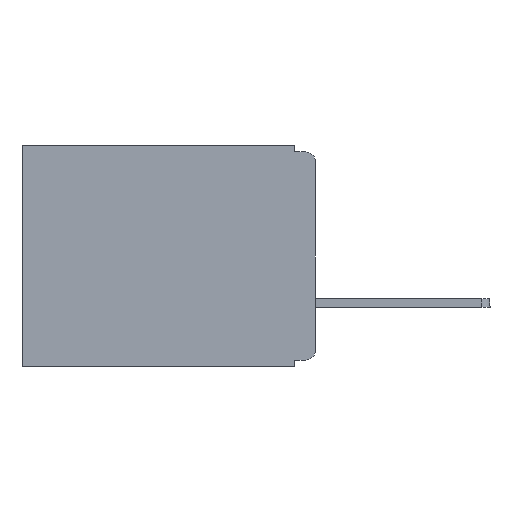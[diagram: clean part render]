
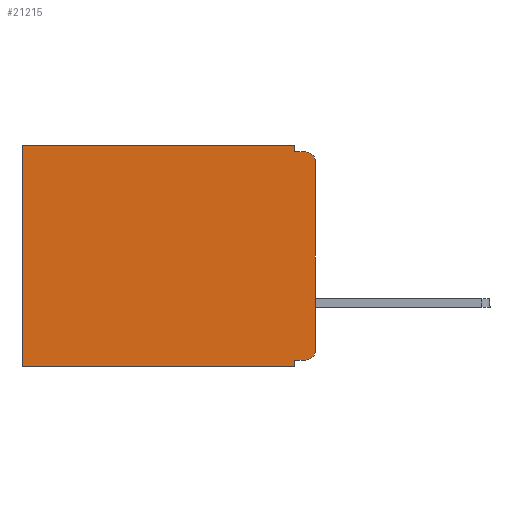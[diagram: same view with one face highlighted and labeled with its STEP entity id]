
A CAD part, left-side view. The second image highlights one B-rep face of the part: STEP entity #21215.
In plain terms, the highlighted planar face has unit normal (-1, 0, 0).
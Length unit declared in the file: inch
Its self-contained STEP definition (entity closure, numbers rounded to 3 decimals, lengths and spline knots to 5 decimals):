
#140 = VECTOR ( 'NONE', #14403, 39.37008 ) ;
#962 = FACE_OUTER_BOUND ( 'NONE', #12624, .T. ) ;
#1121 = VECTOR ( 'NONE', #1252, 39.37008 ) ;
#1252 = DIRECTION ( 'NONE',  ( 0., 0., -1. ) ) ;
#1561 = ORIENTED_EDGE ( 'NONE', *, *, #5486, .F. ) ;
#1730 = CARTESIAN_POINT ( 'NONE',  ( 0.3, 0.031, -0.33 ) ) ;
#2026 = CARTESIAN_POINT ( 'NONE',  ( 0.3, 0.015, -0.305 ) ) ;
#2272 = CARTESIAN_POINT ( 'NONE',  ( 0.3, 0., -0.33 ) ) ;
#2291 = DIRECTION ( 'NONE',  ( 0., 0., -1. ) ) ;
#2718 = CIRCLE ( 'NONE', #22640, 0.015 ) ;
#2800 = CARTESIAN_POINT ( 'NONE',  ( 0.3, 0., -0.33 ) ) ;
#3053 = DIRECTION ( 'NONE',  ( 0., -1., 0. ) ) ;
#3244 = CARTESIAN_POINT ( 'NONE',  ( 0.3, 0., -0.33 ) ) ;
#3465 = ORIENTED_EDGE ( 'NONE', *, *, #17571, .T. ) ;
#3485 = CARTESIAN_POINT ( 'NONE',  ( 0.3, 0.437, -0.33 ) ) ;
#3636 = EDGE_CURVE ( 'NONE', #11892, #8520, #13092, .T. ) ;
#3879 = VERTEX_POINT ( 'NONE', #6805 ) ;
#3928 = ORIENTED_EDGE ( 'NONE', *, *, #9904, .F. ) ;
#3989 = DIRECTION ( 'NONE',  ( 0., 0., -1. ) ) ;
#4638 = EDGE_CURVE ( 'NONE', #15721, #8520, #15747, .T. ) ;
#5136 = CARTESIAN_POINT ( 'NONE',  ( 0.3, 0.031, -0.32 ) ) ;
#5183 = CARTESIAN_POINT ( 'NONE',  ( 0.3, 0.031, -0.01 ) ) ;
#5215 = DIRECTION ( 'NONE',  ( 0., 0., -1. ) ) ;
#5486 = EDGE_CURVE ( 'NONE', #11892, #22754, #9276, .T. ) ;
#5945 = CARTESIAN_POINT ( 'NONE',  ( 0.3, 0.437, -0.33 ) ) ;
#6805 = CARTESIAN_POINT ( 'NONE',  ( 0.3, 0.015, -0.32 ) ) ;
#6896 = VERTEX_POINT ( 'NONE', #5136 ) ;
#6930 = ORIENTED_EDGE ( 'NONE', *, *, #13381, .F. ) ;
#7332 = LINE ( 'NONE', #24920, #17737 ) ;
#7629 = CARTESIAN_POINT ( 'NONE',  ( 0.3, 0.031, 0. ) ) ;
#7677 = CARTESIAN_POINT ( 'NONE',  ( 0.3, 0., -0.01 ) ) ;
#8383 = CARTESIAN_POINT ( 'NONE',  ( 0.3, 0.015, -0.01 ) ) ;
#8484 = AXIS2_PLACEMENT_3D ( 'NONE', #3244, #16938, #5215 ) ;
#8520 = VERTEX_POINT ( 'NONE', #8383 ) ;
#9276 = LINE ( 'NONE', #2272, #14460 ) ;
#9584 = ORIENTED_EDGE ( 'NONE', *, *, #16401, .T. ) ;
#9593 = DIRECTION ( 'NONE',  ( 0., 0., -1. ) ) ;
#9713 = VERTEX_POINT ( 'NONE', #5945 ) ;
#9904 = EDGE_CURVE ( 'NONE', #3879, #6896, #20897, .T. ) ;
#10263 = ORIENTED_EDGE ( 'NONE', *, *, #23991, .F. ) ;
#10330 = VECTOR ( 'NONE', #13284, 39.37008 ) ;
#11076 = ORIENTED_EDGE ( 'NONE', *, *, #4638, .F. ) ;
#11211 = CARTESIAN_POINT ( 'NONE',  ( 0.3, 0.015, -0.025 ) ) ;
#11425 = DIRECTION ( 'NONE',  ( 0., 1., 0. ) ) ;
#11566 = LINE ( 'NONE', #3485, #10330 ) ;
#11892 = VERTEX_POINT ( 'NONE', #17041 ) ;
#12520 = DIRECTION ( 'NONE',  ( -1., 0., 0. ) ) ;
#12586 = DIRECTION ( 'NONE',  ( 0., 0., -1. ) ) ;
#12609 = EDGE_CURVE ( 'NONE', #3879, #22754, #2718, .T. ) ;
#12624 = EDGE_LOOP ( 'NONE', ( #1561, #21098, #11076, #19906, #9584, #3465, #6930, #10263, #3928, #22534 ) ) ;
#13092 = CIRCLE ( 'NONE', #24223, 0.015 ) ;
#13099 = VECTOR ( 'NONE', #9593, 39.37008 ) ;
#13284 = DIRECTION ( 'NONE',  ( 0., 0., -1. ) ) ;
#13357 = LINE ( 'NONE', #7629, #13099 ) ;
#13381 = EDGE_CURVE ( 'NONE', #16997, #9713, #23982, .T. ) ;
#14403 = DIRECTION ( 'NONE',  ( 0., 1., 0. ) ) ;
#14460 = VECTOR ( 'NONE', #2291, 39.37008 ) ;
#14916 = CARTESIAN_POINT ( 'NONE',  ( 0.3, 0.031, -0.33 ) ) ;
#15111 = VECTOR ( 'NONE', #3053, 39.37008 ) ;
#15575 = VERTEX_POINT ( 'NONE', #18424 ) ;
#15692 = DIRECTION ( 'NONE',  ( -1., 0., 0. ) ) ;
#15721 = VERTEX_POINT ( 'NONE', #5183 ) ;
#15747 = LINE ( 'NONE', #7677, #15111 ) ;
#16401 = EDGE_CURVE ( 'NONE', #15575, #21978, #7332, .T. ) ;
#16508 = DIRECTION ( 'NONE',  ( 0., 1., 0. ) ) ;
#16938 = DIRECTION ( 'NONE',  ( 1., 0., 0. ) ) ;
#16997 = VERTEX_POINT ( 'NONE', #1730 ) ;
#17041 = CARTESIAN_POINT ( 'NONE',  ( 0.3, 0., -0.025 ) ) ;
#17571 = EDGE_CURVE ( 'NONE', #21978, #9713, #11566, .T. ) ;
#17737 = VECTOR ( 'NONE', #11425, 39.37008 ) ;
#18424 = CARTESIAN_POINT ( 'NONE',  ( 0.3, 0.031, 0. ) ) ;
#19906 = ORIENTED_EDGE ( 'NONE', *, *, #24731, .F. ) ;
#20082 = VECTOR ( 'NONE', #16508, 39.37008 ) ;
#20897 = LINE ( 'NONE', #24022, #140 ) ;
#21098 = ORIENTED_EDGE ( 'NONE', *, *, #3636, .T. ) ;
#21215 = ADVANCED_FACE ( 'NONE', ( #962 ), #24563, .F. ) ;
#21274 = LINE ( 'NONE', #14916, #1121 ) ;
#21691 = CARTESIAN_POINT ( 'NONE',  ( 0.3, 0., -0.305 ) ) ;
#21978 = VERTEX_POINT ( 'NONE', #23144 ) ;
#22534 = ORIENTED_EDGE ( 'NONE', *, *, #12609, .T. ) ;
#22640 = AXIS2_PLACEMENT_3D ( 'NONE', #2026, #15692, #3989 ) ;
#22754 = VERTEX_POINT ( 'NONE', #21691 ) ;
#23144 = CARTESIAN_POINT ( 'NONE',  ( 0.3, 0.437, 0. ) ) ;
#23982 = LINE ( 'NONE', #2800, #20082 ) ;
#23991 = EDGE_CURVE ( 'NONE', #6896, #16997, #21274, .T. ) ;
#24022 = CARTESIAN_POINT ( 'NONE',  ( 0.3, 0., -0.32 ) ) ;
#24223 = AXIS2_PLACEMENT_3D ( 'NONE', #11211, #12520, #12586 ) ;
#24563 = PLANE ( 'NONE',  #8484 ) ;
#24731 = EDGE_CURVE ( 'NONE', #15575, #15721, #13357, .T. ) ;
#24920 = CARTESIAN_POINT ( 'NONE',  ( 0.3, 0., 0. ) ) ;
